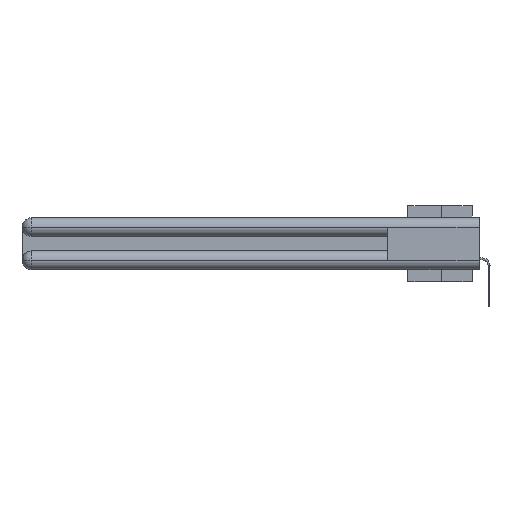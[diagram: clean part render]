
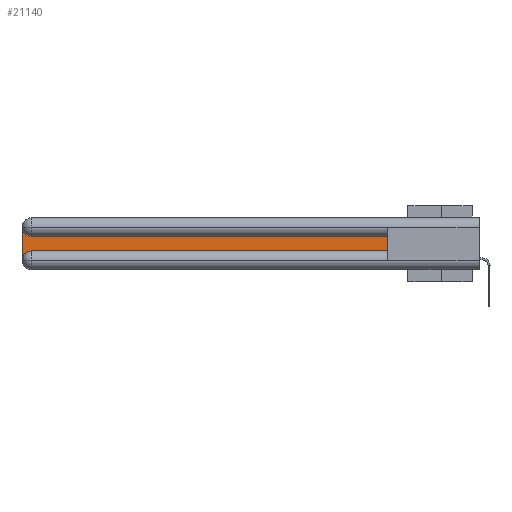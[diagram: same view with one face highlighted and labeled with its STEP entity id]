
A CAD part, left-side view. The second image highlights one B-rep face of the part: STEP entity #21140.
In plain terms, the highlighted planar face has unit normal (-1, 0, 0).
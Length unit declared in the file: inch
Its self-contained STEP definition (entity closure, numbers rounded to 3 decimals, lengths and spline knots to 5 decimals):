
#1779 = DIRECTION ( 'NONE',  ( 0., 1., 0. ) ) ;
#2282 = EDGE_CURVE ( 'NONE', #33847, #20289, #9278, .T. ) ;
#3031 = CARTESIAN_POINT ( 'NONE',  ( 0.075, 2.94, -0.2175 ) ) ;
#3290 = PLANE ( 'NONE',  #10393 ) ;
#3381 = AXIS2_PLACEMENT_3D ( 'NONE', #12862, #26434, #23373 ) ;
#4486 = VECTOR ( 'NONE', #26717, 39.37008 ) ;
#5217 = CARTESIAN_POINT ( 'NONE',  ( 0.075, 0.6, -0.1225 ) ) ;
#5640 = CARTESIAN_POINT ( 'NONE',  ( 0.075, 3., -0.1225 ) ) ;
#5680 = DIRECTION ( 'NONE',  ( 0., 0., -1. ) ) ;
#8690 = AXIS2_PLACEMENT_3D ( 'NONE', #30598, #19527, #22904 ) ;
#9278 = CIRCLE ( 'NONE', #8690, 0.06 ) ;
#10393 = AXIS2_PLACEMENT_3D ( 'NONE', #5640, #13997, #25039 ) ;
#11510 = VECTOR ( 'NONE', #21431, 39.37008 ) ;
#11890 = CARTESIAN_POINT ( 'NONE',  ( 0.075, 2.94, -0.1225 ) ) ;
#11905 = EDGE_CURVE ( 'NONE', #14833, #20241, #13323, .T. ) ;
#12862 = CARTESIAN_POINT ( 'NONE',  ( 0.075, 2.94, -0.0625 ) ) ;
#13027 = CARTESIAN_POINT ( 'NONE',  ( 0.075, 0.6, -0.2175 ) ) ;
#13323 = LINE ( 'NONE', #24367, #4486 ) ;
#13843 = CARTESIAN_POINT ( 'NONE',  ( 0.075, 3., -0.2175 ) ) ;
#13997 = DIRECTION ( 'NONE',  ( 1., 0., 0. ) ) ;
#14346 = ORIENTED_EDGE ( 'NONE', *, *, #18363, .T. ) ;
#14833 = VERTEX_POINT ( 'NONE', #13027 ) ;
#14980 = CIRCLE ( 'NONE', #3381, 0.06 ) ;
#15834 = ORIENTED_EDGE ( 'NONE', *, *, #11905, .T. ) ;
#16553 = LINE ( 'NONE', #13843, #30457 ) ;
#17056 = FACE_OUTER_BOUND ( 'NONE', #17220, .T. ) ;
#17220 = EDGE_LOOP ( 'NONE', ( #22019, #14346, #25399, #25930, #33019, #15834 ) ) ;
#18363 = EDGE_CURVE ( 'NONE', #35629, #28459, #14980, .T. ) ;
#18529 = LINE ( 'NONE', #27225, #11510 ) ;
#19527 = DIRECTION ( 'NONE',  ( 1., 0., 0. ) ) ;
#20241 = VERTEX_POINT ( 'NONE', #22757 ) ;
#20289 = VERTEX_POINT ( 'NONE', #3031 ) ;
#20509 = CARTESIAN_POINT ( 'NONE',  ( 0.075, 3., -0.2775 ) ) ;
#21140 = ADVANCED_FACE ( 'NONE', ( #17056 ), #3290, .F. ) ;
#21431 = DIRECTION ( 'NONE',  ( 0., -1., 0. ) ) ;
#21747 = EDGE_CURVE ( 'NONE', #20241, #35629, #34773, .T. ) ;
#22019 = ORIENTED_EDGE ( 'NONE', *, *, #21747, .T. ) ;
#22757 = CARTESIAN_POINT ( 'NONE',  ( 0.075, 0.6, -0.1225 ) ) ;
#22904 = DIRECTION ( 'NONE',  ( 0., 0., -1. ) ) ;
#23373 = DIRECTION ( 'NONE',  ( 0., 0., -1. ) ) ;
#24367 = CARTESIAN_POINT ( 'NONE',  ( 0.075, 0.6, -0.2175 ) ) ;
#24409 = CARTESIAN_POINT ( 'NONE',  ( 0.075, 3., -0.0625 ) ) ;
#25039 = DIRECTION ( 'NONE',  ( 0., 0., -1. ) ) ;
#25399 = ORIENTED_EDGE ( 'NONE', *, *, #29008, .T. ) ;
#25930 = ORIENTED_EDGE ( 'NONE', *, *, #2282, .T. ) ;
#26434 = DIRECTION ( 'NONE',  ( 1., 0., 0. ) ) ;
#26717 = DIRECTION ( 'NONE',  ( 0., 0., 1. ) ) ;
#27225 = CARTESIAN_POINT ( 'NONE',  ( 0.075, 0.6, -0.2175 ) ) ;
#27788 = VECTOR ( 'NONE', #1779, 39.37008 ) ;
#28459 = VERTEX_POINT ( 'NONE', #24409 ) ;
#29008 = EDGE_CURVE ( 'NONE', #28459, #33847, #16553, .T. ) ;
#30457 = VECTOR ( 'NONE', #5680, 39.37008 ) ;
#30598 = CARTESIAN_POINT ( 'NONE',  ( 0.075, 2.94, -0.2775 ) ) ;
#33019 = ORIENTED_EDGE ( 'NONE', *, *, #33526, .T. ) ;
#33526 = EDGE_CURVE ( 'NONE', #20289, #14833, #18529, .T. ) ;
#33847 = VERTEX_POINT ( 'NONE', #20509 ) ;
#34773 = LINE ( 'NONE', #5217, #27788 ) ;
#35629 = VERTEX_POINT ( 'NONE', #11890 ) ;
